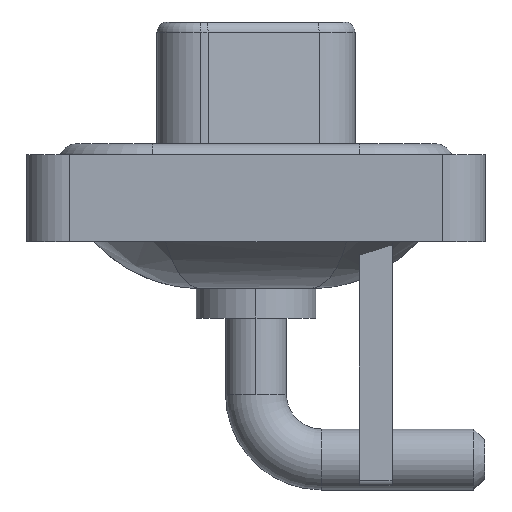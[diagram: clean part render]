
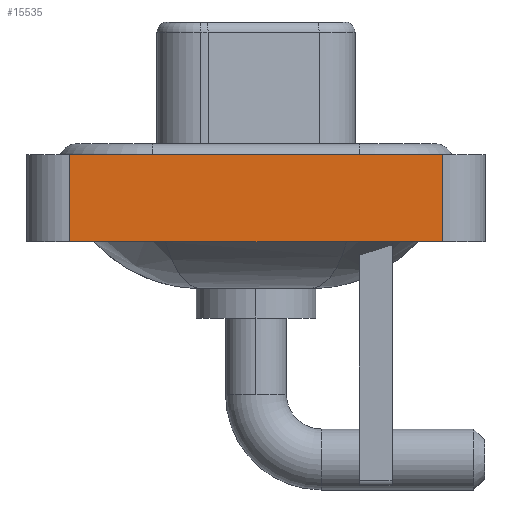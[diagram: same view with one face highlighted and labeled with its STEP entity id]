
A CAD part, left-side view. The second image highlights one B-rep face of the part: STEP entity #15535.
In plain terms, the highlighted planar face has unit normal (-1, 0, 0).
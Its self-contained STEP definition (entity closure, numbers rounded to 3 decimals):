
#169 = CARTESIAN_POINT ( 'NONE',  ( -7.25, -8.55, 0.4 ) ) ;
#354 = CARTESIAN_POINT ( 'NONE',  ( -7.25, 8.55, 0.4 ) ) ;
#1193 = DIRECTION ( 'NONE',  ( 0., -1., 0. ) ) ;
#2061 = ORIENTED_EDGE ( 'NONE', *, *, #4845, .F. ) ;
#2981 = CARTESIAN_POINT ( 'NONE',  ( -7.25, 8.55, -3.6 ) ) ;
#3682 = VECTOR ( 'NONE', #16330, 1000. ) ;
#4017 = CARTESIAN_POINT ( 'NONE',  ( -7.25, -8.55, 0.4 ) ) ;
#4539 = PLANE ( 'NONE',  #14823 ) ;
#4845 = EDGE_CURVE ( 'NONE', #9496, #17700, #12797, .T. ) ;
#4852 = EDGE_CURVE ( 'NONE', #14007, #9496, #5614, .T. ) ;
#5610 = CARTESIAN_POINT ( 'NONE',  ( -7.25, -8.55, -3.6 ) ) ;
#5614 = LINE ( 'NONE', #2981, #13117 ) ;
#6080 = LINE ( 'NONE', #7487, #12861 ) ;
#6226 = EDGE_CURVE ( 'NONE', #9735, #17700, #6080, .T. ) ;
#7487 = CARTESIAN_POINT ( 'NONE',  ( -7.25, -8.55, -3.6 ) ) ;
#8728 = DIRECTION ( 'NONE',  ( 0., 0., 1. ) ) ;
#8786 = CARTESIAN_POINT ( 'NONE',  ( -7.25, -8.55, -3.6 ) ) ;
#9496 = VERTEX_POINT ( 'NONE', #354 ) ;
#9735 = VERTEX_POINT ( 'NONE', #5610 ) ;
#9844 = ORIENTED_EDGE ( 'NONE', *, *, #4852, .F. ) ;
#9943 = DIRECTION ( 'NONE',  ( -1., 0., 0. ) ) ;
#10974 = LINE ( 'NONE', #13703, #3682 ) ;
#11634 = DIRECTION ( 'NONE',  ( 0., 0., 1. ) ) ;
#11945 = DIRECTION ( 'NONE',  ( 0., 0., 1. ) ) ;
#12696 = CARTESIAN_POINT ( 'NONE',  ( -7.25, 8.55, -3.6 ) ) ;
#12797 = LINE ( 'NONE', #4017, #17329 ) ;
#12861 = VECTOR ( 'NONE', #8728, 1000. ) ;
#13117 = VECTOR ( 'NONE', #11945, 1000. ) ;
#13179 = EDGE_LOOP ( 'NONE', ( #13911, #2061, #9844, #17586 ) ) ;
#13703 = CARTESIAN_POINT ( 'NONE',  ( -7.25, -8.55, -3.6 ) ) ;
#13911 = ORIENTED_EDGE ( 'NONE', *, *, #6226, .T. ) ;
#14007 = VERTEX_POINT ( 'NONE', #12696 ) ;
#14805 = EDGE_CURVE ( 'NONE', #14007, #9735, #10974, .T. ) ;
#14823 = AXIS2_PLACEMENT_3D ( 'NONE', #8786, #9943, #11634 ) ;
#15535 = ADVANCED_FACE ( 'NONE', ( #17479 ), #4539, .T. ) ;
#16330 = DIRECTION ( 'NONE',  ( 0., -1., 0. ) ) ;
#17329 = VECTOR ( 'NONE', #1193, 1000. ) ;
#17479 = FACE_OUTER_BOUND ( 'NONE', #13179, .T. ) ;
#17586 = ORIENTED_EDGE ( 'NONE', *, *, #14805, .T. ) ;
#17700 = VERTEX_POINT ( 'NONE', #169 ) ;
